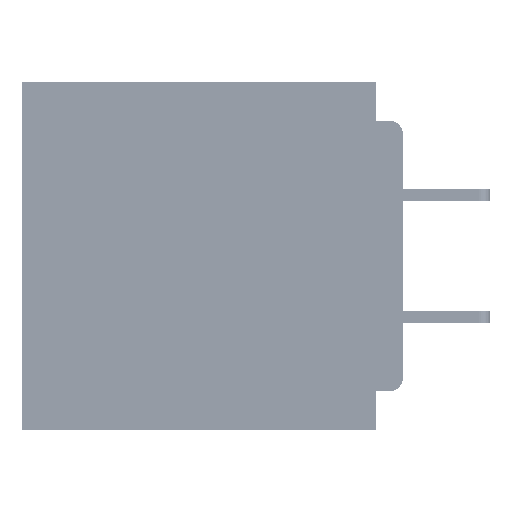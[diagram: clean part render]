
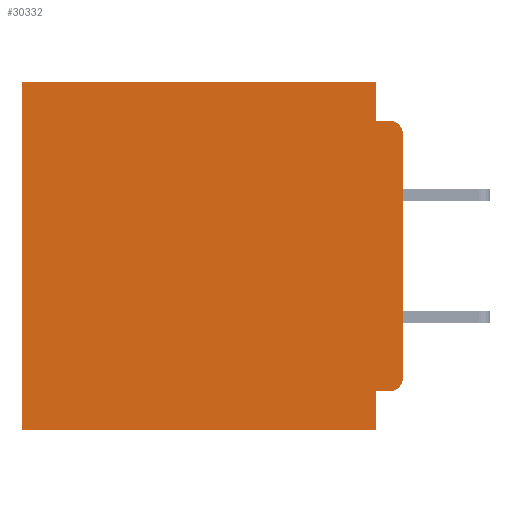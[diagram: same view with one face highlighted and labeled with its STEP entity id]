
A CAD part, left-side view. The second image highlights one B-rep face of the part: STEP entity #30332.
In plain terms, the highlighted planar face has unit normal (-1, 0, 0).
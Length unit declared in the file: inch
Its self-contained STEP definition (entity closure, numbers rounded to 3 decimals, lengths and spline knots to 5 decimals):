
#21 = VERTEX_POINT ( 'NONE', #56206 ) ;
#223 = ORIENTED_EDGE ( 'NONE', *, *, #63342, .F. ) ;
#502 = EDGE_CURVE ( 'NONE', #5982, #13950, #29373, .T. ) ;
#1247 = VERTEX_POINT ( 'NONE', #63694 ) ;
#1474 = CARTESIAN_POINT ( 'NONE',  ( 0.3, 0., -0.4 ) ) ;
#3329 = EDGE_CURVE ( 'NONE', #1247, #13950, #41715, .T. ) ;
#3660 = DIRECTION ( 'NONE',  ( 0., 0., -1. ) ) ;
#5982 = VERTEX_POINT ( 'NONE', #58374 ) ;
#6165 = DIRECTION ( 'NONE',  ( 0., 1., 0. ) ) ;
#7213 = ORIENTED_EDGE ( 'NONE', *, *, #39831, .T. ) ;
#8364 = CARTESIAN_POINT ( 'NONE',  ( 0.3, 0.437, -0.4 ) ) ;
#12008 = DIRECTION ( 'NONE',  ( 0., -1., 0. ) ) ;
#12396 = CARTESIAN_POINT ( 'NONE',  ( 0.3, 0.015, -0.355 ) ) ;
#12455 = ORIENTED_EDGE ( 'NONE', *, *, #3329, .T. ) ;
#13485 = CARTESIAN_POINT ( 'NONE',  ( 0.3, 0.437, 0. ) ) ;
#13950 = VERTEX_POINT ( 'NONE', #37403 ) ;
#13975 = PLANE ( 'NONE',  #17487 ) ;
#14546 = VERTEX_POINT ( 'NONE', #26652 ) ;
#15487 = CARTESIAN_POINT ( 'NONE',  ( 0.3, 0., -0.4 ) ) ;
#17230 = LINE ( 'NONE', #54076, #46577 ) ;
#17487 = AXIS2_PLACEMENT_3D ( 'NONE', #66280, #34894, #3660 ) ;
#17608 = ORIENTED_EDGE ( 'NONE', *, *, #44843, .F. ) ;
#17641 = EDGE_CURVE ( 'NONE', #31982, #14546, #57337, .T. ) ;
#18527 = CARTESIAN_POINT ( 'NONE',  ( 0.3, 0.031, -0.355 ) ) ;
#23873 = LINE ( 'NONE', #58217, #65621 ) ;
#26652 = CARTESIAN_POINT ( 'NONE',  ( 0.3, 0., -0.34 ) ) ;
#27020 = EDGE_LOOP ( 'NONE', ( #223, #12455, #40334, #45368, #7213, #29851, #28316, #17608, #58299, #44762 ) ) ;
#28316 = ORIENTED_EDGE ( 'NONE', *, *, #63176, .F. ) ;
#29373 = LINE ( 'NONE', #41709, #58789 ) ;
#29851 = ORIENTED_EDGE ( 'NONE', *, *, #32856, .T. ) ;
#30332 = ADVANCED_FACE ( 'NONE', ( #58838 ), #13975, .F. ) ;
#30552 = CARTESIAN_POINT ( 'NONE',  ( 0.3, 0.015, -0.34 ) ) ;
#30826 = VECTOR ( 'NONE', #61770, 39.37008 ) ;
#30875 = AXIS2_PLACEMENT_3D ( 'NONE', #30552, #67156, #35769 ) ;
#31818 = LINE ( 'NONE', #15487, #44040 ) ;
#31982 = VERTEX_POINT ( 'NONE', #12396 ) ;
#32419 = LINE ( 'NONE', #51242, #30826 ) ;
#32856 = EDGE_CURVE ( 'NONE', #47537, #21, #35400, .T. ) ;
#33740 = VECTOR ( 'NONE', #39574, 39.37008 ) ;
#33813 = VERTEX_POINT ( 'NONE', #58479 ) ;
#34894 = DIRECTION ( 'NONE',  ( 1., 0., 0. ) ) ;
#35400 = LINE ( 'NONE', #8364, #33740 ) ;
#35769 = DIRECTION ( 'NONE',  ( 0., 0., -1. ) ) ;
#37403 = CARTESIAN_POINT ( 'NONE',  ( 0.3, 0.015, -0.045 ) ) ;
#39442 = VECTOR ( 'NONE', #64734, 39.37008 ) ;
#39574 = DIRECTION ( 'NONE',  ( 0., 0., -1. ) ) ;
#39831 = EDGE_CURVE ( 'NONE', #33813, #47537, #23873, .T. ) ;
#40334 = ORIENTED_EDGE ( 'NONE', *, *, #502, .F. ) ;
#41709 = CARTESIAN_POINT ( 'NONE',  ( 0.3, 0., -0.045 ) ) ;
#41715 = CIRCLE ( 'NONE', #65440, 0.015 ) ;
#42186 = DIRECTION ( 'NONE',  ( 0., 0., -1. ) ) ;
#42275 = DIRECTION ( 'NONE',  ( -1., 0., 0. ) ) ;
#43012 = DIRECTION ( 'NONE',  ( 0., 0., -1. ) ) ;
#43394 = EDGE_CURVE ( 'NONE', #33813, #5982, #61809, .T. ) ;
#43482 = VERTEX_POINT ( 'NONE', #18527 ) ;
#43851 = CARTESIAN_POINT ( 'NONE',  ( 0.3, 0.031, 0. ) ) ;
#44040 = VECTOR ( 'NONE', #46901, 39.37008 ) ;
#44762 = ORIENTED_EDGE ( 'NONE', *, *, #17641, .T. ) ;
#44843 = EDGE_CURVE ( 'NONE', #43482, #45861, #17230, .T. ) ;
#45368 = ORIENTED_EDGE ( 'NONE', *, *, #43394, .F. ) ;
#45861 = VERTEX_POINT ( 'NONE', #62703 ) ;
#46577 = VECTOR ( 'NONE', #49055, 39.37008 ) ;
#46901 = DIRECTION ( 'NONE',  ( 0., 1., 0. ) ) ;
#47537 = VERTEX_POINT ( 'NONE', #13485 ) ;
#49055 = DIRECTION ( 'NONE',  ( 0., 0., -1. ) ) ;
#49172 = CARTESIAN_POINT ( 'NONE',  ( 0.3, 0.015, -0.06 ) ) ;
#51242 = CARTESIAN_POINT ( 'NONE',  ( 0.3, 0., -0.355 ) ) ;
#54076 = CARTESIAN_POINT ( 'NONE',  ( 0.3, 0.031, -0.4 ) ) ;
#56206 = CARTESIAN_POINT ( 'NONE',  ( 0.3, 0.437, -0.4 ) ) ;
#57337 = CIRCLE ( 'NONE', #30875, 0.015 ) ;
#58217 = CARTESIAN_POINT ( 'NONE',  ( 0.3, 0., 0. ) ) ;
#58299 = ORIENTED_EDGE ( 'NONE', *, *, #65442, .F. ) ;
#58374 = CARTESIAN_POINT ( 'NONE',  ( 0.3, 0.031, -0.045 ) ) ;
#58479 = CARTESIAN_POINT ( 'NONE',  ( 0.3, 0.031, 0. ) ) ;
#58789 = VECTOR ( 'NONE', #12008, 39.37008 ) ;
#58838 = FACE_OUTER_BOUND ( 'NONE', #27020, .T. ) ;
#61770 = DIRECTION ( 'NONE',  ( 0., 1., 0. ) ) ;
#61809 = LINE ( 'NONE', #43851, #39442 ) ;
#62097 = VECTOR ( 'NONE', #43012, 39.37008 ) ;
#62703 = CARTESIAN_POINT ( 'NONE',  ( 0.3, 0.031, -0.4 ) ) ;
#63176 = EDGE_CURVE ( 'NONE', #45861, #21, #31818, .T. ) ;
#63342 = EDGE_CURVE ( 'NONE', #1247, #14546, #63746, .T. ) ;
#63694 = CARTESIAN_POINT ( 'NONE',  ( 0.3, 0., -0.06 ) ) ;
#63746 = LINE ( 'NONE', #1474, #62097 ) ;
#64734 = DIRECTION ( 'NONE',  ( 0., 0., -1. ) ) ;
#65440 = AXIS2_PLACEMENT_3D ( 'NONE', #49172, #42275, #42186 ) ;
#65442 = EDGE_CURVE ( 'NONE', #31982, #43482, #32419, .T. ) ;
#65621 = VECTOR ( 'NONE', #6165, 39.37008 ) ;
#66280 = CARTESIAN_POINT ( 'NONE',  ( 0.3, 0., -0.4 ) ) ;
#67156 = DIRECTION ( 'NONE',  ( -1., 0., 0. ) ) ;
